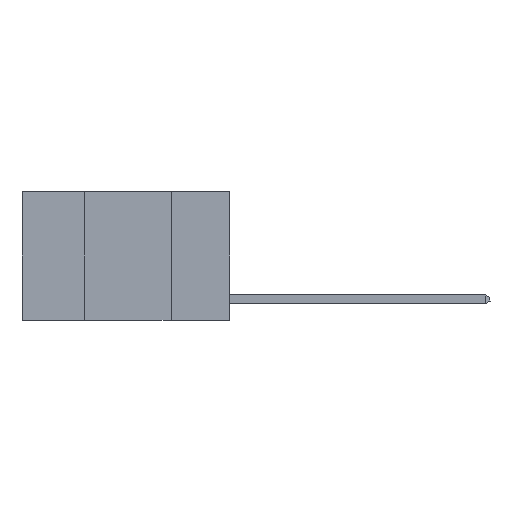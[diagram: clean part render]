
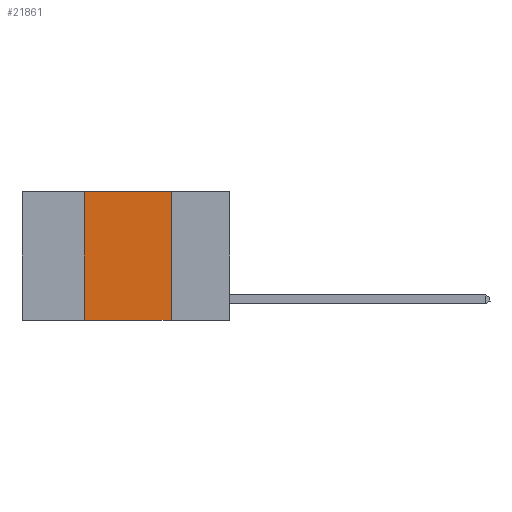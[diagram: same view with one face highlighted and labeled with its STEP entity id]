
A CAD part, left-side view. The second image highlights one B-rep face of the part: STEP entity #21861.
In plain terms, the highlighted planar face has unit normal (-1, 0, 0).
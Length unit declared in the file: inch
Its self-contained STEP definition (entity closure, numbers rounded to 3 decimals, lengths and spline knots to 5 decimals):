
#1719 = CARTESIAN_POINT ( 'NONE',  ( 0., 0.42, 0. ) ) ;
#1762 = DIRECTION ( 'NONE',  ( 0., -1., 0. ) ) ;
#2036 = VECTOR ( 'NONE', #20123, 39.37008 ) ;
#3036 = EDGE_CURVE ( 'NONE', #21001, #6082, #3609, .T. ) ;
#3609 = LINE ( 'NONE', #20259, #6827 ) ;
#4252 = EDGE_CURVE ( 'NONE', #21001, #16126, #11920, .T. ) ;
#4341 = ORIENTED_EDGE ( 'NONE', *, *, #16118, .F. ) ;
#4365 = ORIENTED_EDGE ( 'NONE', *, *, #21021, .F. ) ;
#4544 = ORIENTED_EDGE ( 'NONE', *, *, #4252, .F. ) ;
#5030 = ORIENTED_EDGE ( 'NONE', *, *, #3036, .T. ) ;
#5208 = VERTEX_POINT ( 'NONE', #9120 ) ;
#6082 = VERTEX_POINT ( 'NONE', #11732 ) ;
#6827 = VECTOR ( 'NONE', #1762, 39.37008 ) ;
#8228 = DIRECTION ( 'NONE',  ( 1., 0., 0. ) ) ;
#8449 = CARTESIAN_POINT ( 'NONE',  ( 0., 0.17, 0. ) ) ;
#9120 = CARTESIAN_POINT ( 'NONE',  ( 0., 0.17, 0. ) ) ;
#9255 = DIRECTION ( 'NONE',  ( 0., -1., 0. ) ) ;
#10464 = LINE ( 'NONE', #11103, #23393 ) ;
#11103 = CARTESIAN_POINT ( 'NONE',  ( 0., 0.6, 0. ) ) ;
#11732 = CARTESIAN_POINT ( 'NONE',  ( 0., 0.17, -0.37 ) ) ;
#11920 = LINE ( 'NONE', #1719, #2036 ) ;
#12078 = LINE ( 'NONE', #8449, #16447 ) ;
#12142 = DIRECTION ( 'NONE',  ( 0., 0., -1. ) ) ;
#14003 = CARTESIAN_POINT ( 'NONE',  ( 0., 0.42, 0. ) ) ;
#14897 = EDGE_LOOP ( 'NONE', ( #4341, #4365, #4544, #5030 ) ) ;
#15566 = CARTESIAN_POINT ( 'NONE',  ( 0., 0.6, 0. ) ) ;
#16118 = EDGE_CURVE ( 'NONE', #5208, #6082, #12078, .T. ) ;
#16126 = VERTEX_POINT ( 'NONE', #14003 ) ;
#16447 = VECTOR ( 'NONE', #12142, 39.37008 ) ;
#16585 = CARTESIAN_POINT ( 'NONE',  ( 0., 0.42, -0.37 ) ) ;
#19308 = PLANE ( 'NONE',  #21114 ) ;
#19644 = FACE_OUTER_BOUND ( 'NONE', #14897, .T. ) ;
#20123 = DIRECTION ( 'NONE',  ( 0., 0., 1. ) ) ;
#20259 = CARTESIAN_POINT ( 'NONE',  ( 0., 0.6, -0.37 ) ) ;
#21001 = VERTEX_POINT ( 'NONE', #16585 ) ;
#21021 = EDGE_CURVE ( 'NONE', #16126, #5208, #10464, .T. ) ;
#21114 = AXIS2_PLACEMENT_3D ( 'NONE', #15566, #8228, #21130 ) ;
#21130 = DIRECTION ( 'NONE',  ( 0., 0., -1. ) ) ;
#21861 = ADVANCED_FACE ( 'NONE', ( #19644 ), #19308, .F. ) ;
#23393 = VECTOR ( 'NONE', #9255, 39.37008 ) ;
